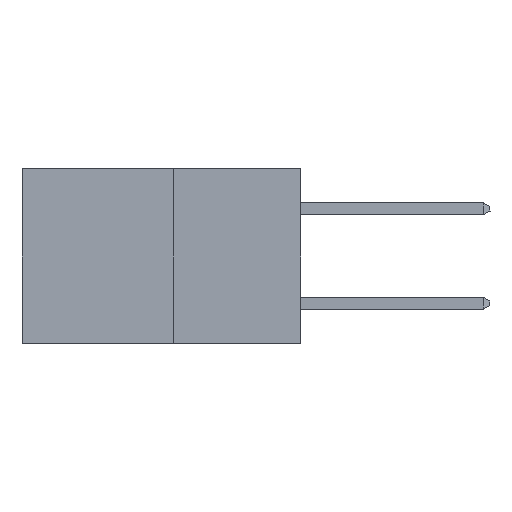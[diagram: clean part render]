
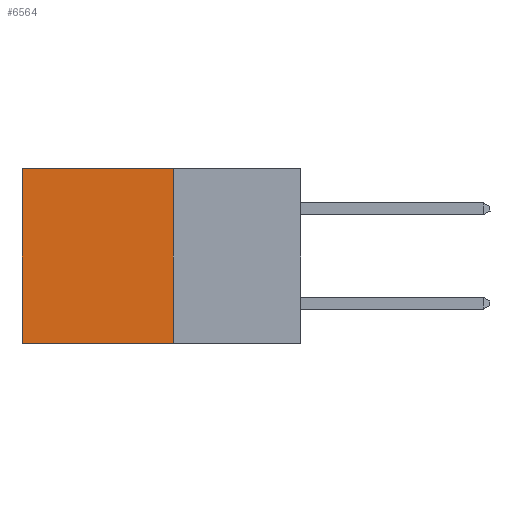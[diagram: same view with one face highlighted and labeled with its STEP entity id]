
A CAD part, left-side view. The second image highlights one B-rep face of the part: STEP entity #6564.
In plain terms, the highlighted planar face has unit normal (-1, 0, 0).
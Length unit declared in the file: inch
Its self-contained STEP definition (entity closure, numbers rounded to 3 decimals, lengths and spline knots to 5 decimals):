
#221 = DIRECTION ( 'NONE',  ( 0., 1., 0. ) ) ;
#253 = FACE_OUTER_BOUND ( 'NONE', #8056, .T. ) ;
#960 = LINE ( 'NONE', #5832, #5670 ) ;
#1913 = VERTEX_POINT ( 'NONE', #4576 ) ;
#2724 = VECTOR ( 'NONE', #221, 39.37008 ) ;
#2958 = CARTESIAN_POINT ( 'NONE',  ( 0.277, 0.27, -0.37 ) ) ;
#2978 = DIRECTION ( 'NONE',  ( 0., 1., 0. ) ) ;
#2996 = ORIENTED_EDGE ( 'NONE', *, *, #11765, .T. ) ;
#3132 = ORIENTED_EDGE ( 'NONE', *, *, #5636, .F. ) ;
#4576 = CARTESIAN_POINT ( 'NONE',  ( 0.277, 0.27, 0. ) ) ;
#4644 = CARTESIAN_POINT ( 'NONE',  ( 0.277, 0.59, 0. ) ) ;
#4905 = EDGE_CURVE ( 'NONE', #1913, #15117, #8487, .T. ) ;
#5636 = EDGE_CURVE ( 'NONE', #15117, #14567, #20697, .T. ) ;
#5670 = VECTOR ( 'NONE', #21547, 39.37008 ) ;
#5832 = CARTESIAN_POINT ( 'NONE',  ( 0.277, 0.59, -0.37 ) ) ;
#6564 = ADVANCED_FACE ( 'NONE', ( #253 ), #24248, .F. ) ;
#7050 = ORIENTED_EDGE ( 'NONE', *, *, #4905, .F. ) ;
#8056 = EDGE_LOOP ( 'NONE', ( #19229, #3132, #7050, #2996 ) ) ;
#8487 = LINE ( 'NONE', #11751, #12541 ) ;
#10943 = VECTOR ( 'NONE', #2978, 39.37008 ) ;
#11751 = CARTESIAN_POINT ( 'NONE',  ( 0.277, 0.27, -0.37 ) ) ;
#11765 = EDGE_CURVE ( 'NONE', #1913, #15879, #13347, .T. ) ;
#12541 = VECTOR ( 'NONE', #14857, 39.37008 ) ;
#13347 = LINE ( 'NONE', #23838, #2724 ) ;
#14567 = VERTEX_POINT ( 'NONE', #20039 ) ;
#14857 = DIRECTION ( 'NONE',  ( 0., 0., -1. ) ) ;
#15117 = VERTEX_POINT ( 'NONE', #15938 ) ;
#15879 = VERTEX_POINT ( 'NONE', #4644 ) ;
#15938 = CARTESIAN_POINT ( 'NONE',  ( 0.277, 0.27, -0.37 ) ) ;
#19229 = ORIENTED_EDGE ( 'NONE', *, *, #19305, .T. ) ;
#19305 = EDGE_CURVE ( 'NONE', #15879, #14567, #960, .T. ) ;
#20030 = AXIS2_PLACEMENT_3D ( 'NONE', #24428, #23684, #23653 ) ;
#20039 = CARTESIAN_POINT ( 'NONE',  ( 0.277, 0.59, -0.37 ) ) ;
#20697 = LINE ( 'NONE', #2958, #10943 ) ;
#21547 = DIRECTION ( 'NONE',  ( 0., 0., -1. ) ) ;
#23653 = DIRECTION ( 'NONE',  ( 0., 0., -1. ) ) ;
#23684 = DIRECTION ( 'NONE',  ( 1., 0., 0. ) ) ;
#23838 = CARTESIAN_POINT ( 'NONE',  ( 0.277, 0.27, 0. ) ) ;
#24248 = PLANE ( 'NONE',  #20030 ) ;
#24428 = CARTESIAN_POINT ( 'NONE',  ( 0.277, 0.27, -0.37 ) ) ;
